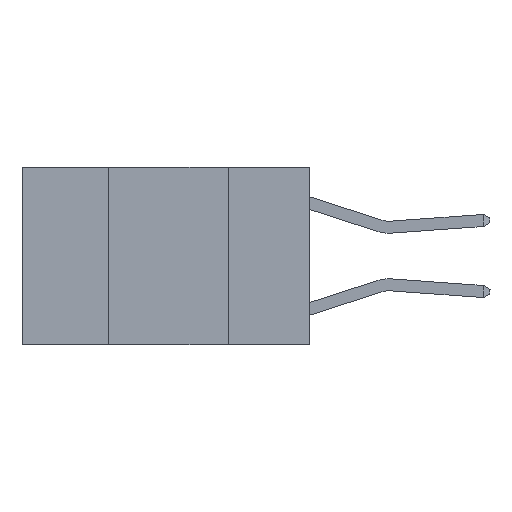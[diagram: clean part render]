
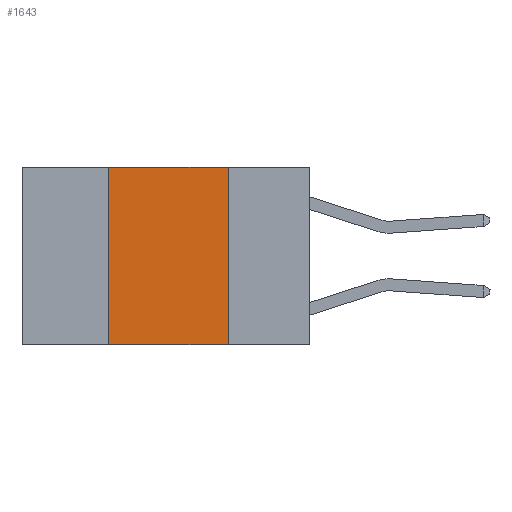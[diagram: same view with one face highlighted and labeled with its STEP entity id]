
A CAD part, left-side view. The second image highlights one B-rep face of the part: STEP entity #1643.
In plain terms, the highlighted planar face has unit normal (-1, 0, 0).
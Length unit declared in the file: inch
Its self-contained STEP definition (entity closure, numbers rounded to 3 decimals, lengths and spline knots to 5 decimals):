
#1643 = ADVANCED_FACE ( 'NONE', ( #15647 ), #29534, .F. ) ;
#1676 = CARTESIAN_POINT ( 'NONE',  ( 0., 0.6, -0.37 ) ) ;
#2291 = CARTESIAN_POINT ( 'NONE',  ( 0., 0.42, -0.37 ) ) ;
#2650 = VERTEX_POINT ( 'NONE', #2291 ) ;
#2864 = CARTESIAN_POINT ( 'NONE',  ( 0., 0.17, 0. ) ) ;
#3113 = CARTESIAN_POINT ( 'NONE',  ( 0., 0.42, 0. ) ) ;
#4168 = DIRECTION ( 'NONE',  ( 0., -1., 0. ) ) ;
#4234 = VERTEX_POINT ( 'NONE', #2864 ) ;
#4632 = LINE ( 'NONE', #26571, #16808 ) ;
#5250 = ORIENTED_EDGE ( 'NONE', *, *, #7402, .F. ) ;
#5348 = LINE ( 'NONE', #1676, #11068 ) ;
#6027 = ORIENTED_EDGE ( 'NONE', *, *, #23580, .F. ) ;
#7402 = EDGE_CURVE ( 'NONE', #24054, #4234, #10961, .T. ) ;
#10404 = DIRECTION ( 'NONE',  ( 0., 0., -1. ) ) ;
#10961 = LINE ( 'NONE', #25651, #30884 ) ;
#11068 = VECTOR ( 'NONE', #4168, 39.37008 ) ;
#12067 = VERTEX_POINT ( 'NONE', #29303 ) ;
#12455 = EDGE_CURVE ( 'NONE', #2650, #12067, #5348, .T. ) ;
#15647 = FACE_OUTER_BOUND ( 'NONE', #16021, .T. ) ;
#15949 = CARTESIAN_POINT ( 'NONE',  ( 0., 0.17, 0. ) ) ;
#16021 = EDGE_LOOP ( 'NONE', ( #6027, #5250, #23789, #16672 ) ) ;
#16672 = ORIENTED_EDGE ( 'NONE', *, *, #12455, .T. ) ;
#16808 = VECTOR ( 'NONE', #28978, 39.37008 ) ;
#18458 = DIRECTION ( 'NONE',  ( 0., 0., -1. ) ) ;
#21377 = VECTOR ( 'NONE', #18458, 39.37008 ) ;
#22114 = LINE ( 'NONE', #15949, #21377 ) ;
#23580 = EDGE_CURVE ( 'NONE', #4234, #12067, #22114, .T. ) ;
#23789 = ORIENTED_EDGE ( 'NONE', *, *, #25370, .F. ) ;
#24054 = VERTEX_POINT ( 'NONE', #3113 ) ;
#25370 = EDGE_CURVE ( 'NONE', #2650, #24054, #4632, .T. ) ;
#25651 = CARTESIAN_POINT ( 'NONE',  ( 0., 0.6, 0. ) ) ;
#26571 = CARTESIAN_POINT ( 'NONE',  ( 0., 0.42, 0. ) ) ;
#26861 = DIRECTION ( 'NONE',  ( 1., 0., 0. ) ) ;
#28053 = DIRECTION ( 'NONE',  ( 0., -1., 0. ) ) ;
#28860 = CARTESIAN_POINT ( 'NONE',  ( 0., 0.6, 0. ) ) ;
#28978 = DIRECTION ( 'NONE',  ( 0., 0., 1. ) ) ;
#29303 = CARTESIAN_POINT ( 'NONE',  ( 0., 0.17, -0.37 ) ) ;
#29534 = PLANE ( 'NONE',  #30049 ) ;
#30049 = AXIS2_PLACEMENT_3D ( 'NONE', #28860, #26861, #10404 ) ;
#30884 = VECTOR ( 'NONE', #28053, 39.37008 ) ;
